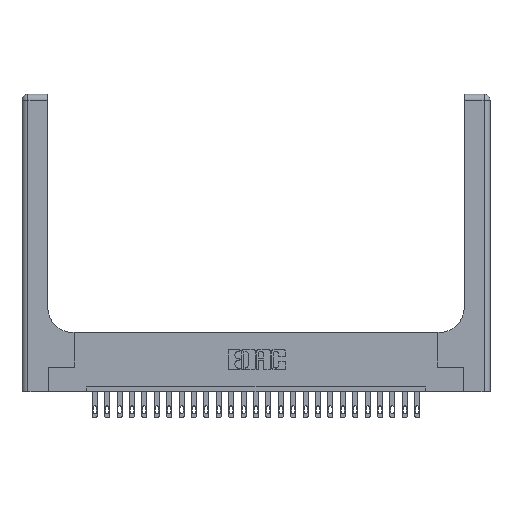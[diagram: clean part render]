
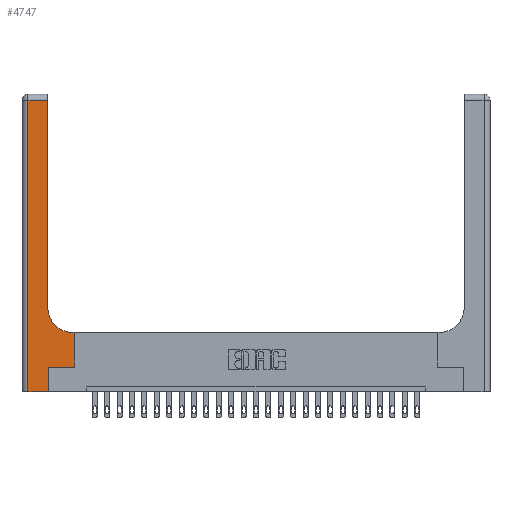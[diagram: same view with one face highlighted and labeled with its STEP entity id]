
A CAD part, top view. The second image highlights one B-rep face of the part: STEP entity #4747.
In plain terms, the highlighted planar face has unit normal (0, 0, 1).
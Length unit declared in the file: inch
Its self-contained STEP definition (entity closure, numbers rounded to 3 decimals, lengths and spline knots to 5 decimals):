
#243 = CARTESIAN_POINT ( 'NONE',  ( 0.26, 3., 0.37 ) ) ;
#530 = DIRECTION ( 'NONE',  ( 0., 1., 0. ) ) ;
#1302 = EDGE_CURVE ( 'NONE', #4836, #6103, #15312, .T. ) ;
#1477 = DIRECTION ( 'NONE',  ( 1., 0., 0. ) ) ;
#1749 = AXIS2_PLACEMENT_3D ( 'NONE', #17821, #21633, #6655 ) ;
#2136 = ORIENTED_EDGE ( 'NONE', *, *, #18621, .T. ) ;
#2421 = CARTESIAN_POINT ( 'NONE',  ( 0.51, 0.6, 0.37 ) ) ;
#2466 = VERTEX_POINT ( 'NONE', #8878 ) ;
#2606 = ORIENTED_EDGE ( 'NONE', *, *, #10346, .T. ) ;
#2783 = LINE ( 'NONE', #15576, #9733 ) ;
#2945 = CARTESIAN_POINT ( 'NONE',  ( 0.528, 0.6, 0.37 ) ) ;
#4017 = CARTESIAN_POINT ( 'NONE',  ( 0., 2.94, 0.37 ) ) ;
#4181 = DIRECTION ( 'NONE',  ( 1., 0., 0. ) ) ;
#4687 = VERTEX_POINT ( 'NONE', #9616 ) ;
#4747 = ADVANCED_FACE ( 'NONE', ( #17944 ), #12200, .F. ) ;
#4836 = VERTEX_POINT ( 'NONE', #2945 ) ;
#4940 = CARTESIAN_POINT ( 'NONE',  ( 0.06, 3., 0.37 ) ) ;
#5122 = EDGE_CURVE ( 'NONE', #4687, #2466, #20998, .T. ) ;
#5533 = ORIENTED_EDGE ( 'NONE', *, *, #15605, .T. ) ;
#5826 = CARTESIAN_POINT ( 'NONE',  ( 0.265, 0., 0.37 ) ) ;
#6040 = LINE ( 'NONE', #243, #17046 ) ;
#6103 = VERTEX_POINT ( 'NONE', #2421 ) ;
#6217 = CARTESIAN_POINT ( 'NONE',  ( 0.26, 0.6, 0.37 ) ) ;
#6557 = CARTESIAN_POINT ( 'NONE',  ( 0.06, 2.94, 0.37 ) ) ;
#6655 = DIRECTION ( 'NONE',  ( -1., 0., 0. ) ) ;
#7234 = VERTEX_POINT ( 'NONE', #24010 ) ;
#7271 = CARTESIAN_POINT ( 'NONE',  ( 0., 0., 0.37 ) ) ;
#7482 = VECTOR ( 'NONE', #16245, 39.37008 ) ;
#7857 = VERTEX_POINT ( 'NONE', #11778 ) ;
#8444 = VECTOR ( 'NONE', #4181, 39.37008 ) ;
#8568 = DIRECTION ( 'NONE',  ( 1., 0., 0. ) ) ;
#8816 = VECTOR ( 'NONE', #1477, 39.37008 ) ;
#8878 = CARTESIAN_POINT ( 'NONE',  ( 0.528, 0.25, 0.37 ) ) ;
#9409 = ORIENTED_EDGE ( 'NONE', *, *, #16838, .T. ) ;
#9616 = CARTESIAN_POINT ( 'NONE',  ( 0.265, 0.25, 0.37 ) ) ;
#9668 = DIRECTION ( 'NONE',  ( -1., 0., 0. ) ) ;
#9733 = VECTOR ( 'NONE', #19508, 39.37008 ) ;
#10346 = EDGE_CURVE ( 'NONE', #6103, #7857, #23970, .T. ) ;
#11196 = LINE ( 'NONE', #7271, #8816 ) ;
#11552 = CARTESIAN_POINT ( 'NONE',  ( 0.265, 0.25, 0.37 ) ) ;
#11778 = CARTESIAN_POINT ( 'NONE',  ( 0.26, 0.85, 0.37 ) ) ;
#12200 = PLANE ( 'NONE',  #1749 ) ;
#12260 = CARTESIAN_POINT ( 'NONE',  ( 0.51, 0.85, 0.37 ) ) ;
#12444 = VECTOR ( 'NONE', #13344, 39.37008 ) ;
#13344 = DIRECTION ( 'NONE',  ( -1., 0., 0. ) ) ;
#13611 = ORIENTED_EDGE ( 'NONE', *, *, #1302, .T. ) ;
#14673 = CARTESIAN_POINT ( 'NONE',  ( 0.26, 2.94, 0.37 ) ) ;
#14742 = EDGE_CURVE ( 'NONE', #24271, #4687, #15178, .T. ) ;
#15092 = ORIENTED_EDGE ( 'NONE', *, *, #22599, .T. ) ;
#15178 = LINE ( 'NONE', #19114, #15398 ) ;
#15312 = LINE ( 'NONE', #6217, #18816 ) ;
#15398 = VECTOR ( 'NONE', #530, 39.37008 ) ;
#15576 = CARTESIAN_POINT ( 'NONE',  ( 0.528, 0.25, 0.37 ) ) ;
#15605 = EDGE_CURVE ( 'NONE', #2466, #4836, #2783, .T. ) ;
#16111 = EDGE_LOOP ( 'NONE', ( #9409, #15092, #2136, #16491, #22058, #19963, #5533, #13611, #2606 ) ) ;
#16245 = DIRECTION ( 'NONE',  ( 0., -1., 0. ) ) ;
#16491 = ORIENTED_EDGE ( 'NONE', *, *, #21494, .T. ) ;
#16838 = EDGE_CURVE ( 'NONE', #7857, #21024, #6040, .T. ) ;
#17046 = VECTOR ( 'NONE', #19764, 39.37008 ) ;
#17673 = AXIS2_PLACEMENT_3D ( 'NONE', #12260, #19735, #8568 ) ;
#17821 = CARTESIAN_POINT ( 'NONE',  ( 0., 3., 0.37 ) ) ;
#17944 = FACE_OUTER_BOUND ( 'NONE', #16111, .T. ) ;
#18621 = EDGE_CURVE ( 'NONE', #19860, #7234, #24218, .T. ) ;
#18643 = LINE ( 'NONE', #4017, #12444 ) ;
#18816 = VECTOR ( 'NONE', #9668, 39.37008 ) ;
#19114 = CARTESIAN_POINT ( 'NONE',  ( 0.265, 0., 0.37 ) ) ;
#19508 = DIRECTION ( 'NONE',  ( 0., 1., 0. ) ) ;
#19735 = DIRECTION ( 'NONE',  ( 0., 0., -1. ) ) ;
#19764 = DIRECTION ( 'NONE',  ( 0., 1., 0. ) ) ;
#19860 = VERTEX_POINT ( 'NONE', #6557 ) ;
#19963 = ORIENTED_EDGE ( 'NONE', *, *, #5122, .T. ) ;
#20998 = LINE ( 'NONE', #11552, #8444 ) ;
#21024 = VERTEX_POINT ( 'NONE', #14673 ) ;
#21494 = EDGE_CURVE ( 'NONE', #7234, #24271, #11196, .T. ) ;
#21633 = DIRECTION ( 'NONE',  ( 0., 0., -1. ) ) ;
#22058 = ORIENTED_EDGE ( 'NONE', *, *, #14742, .T. ) ;
#22599 = EDGE_CURVE ( 'NONE', #21024, #19860, #18643, .T. ) ;
#23970 = CIRCLE ( 'NONE', #17673, 0.25 ) ;
#24010 = CARTESIAN_POINT ( 'NONE',  ( 0.06, 0., 0.37 ) ) ;
#24218 = LINE ( 'NONE', #4940, #7482 ) ;
#24271 = VERTEX_POINT ( 'NONE', #5826 ) ;
